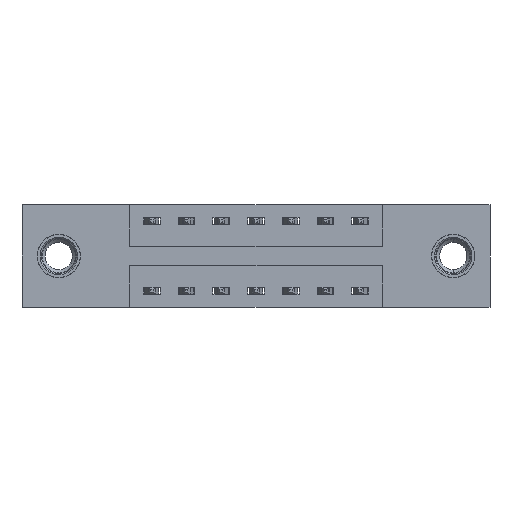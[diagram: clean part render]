
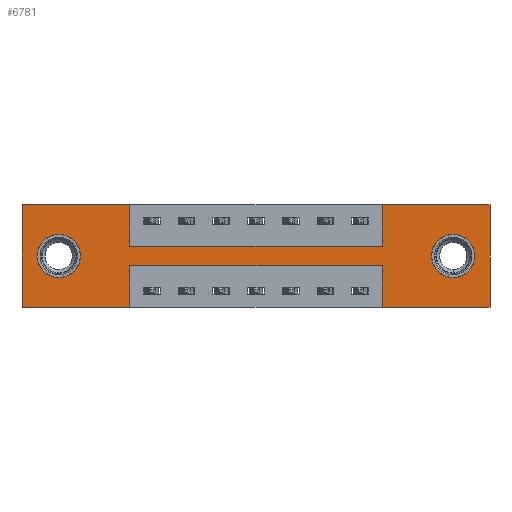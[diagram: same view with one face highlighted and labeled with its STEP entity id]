
A CAD part, front view. The second image highlights one B-rep face of the part: STEP entity #6781.
In plain terms, the highlighted planar face has unit normal (0, -1, 0).
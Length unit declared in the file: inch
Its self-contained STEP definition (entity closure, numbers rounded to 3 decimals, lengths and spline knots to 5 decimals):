
#21 = ORIENTED_EDGE ( 'NONE', *, *, #8824, .F. ) ;
#63 = VERTEX_POINT ( 'NONE', #7902 ) ;
#64 = LINE ( 'NONE', #4035, #4696 ) ;
#182 = CARTESIAN_POINT ( 'NONE',  ( 1.685, 0., 0. ) ) ;
#253 = CARTESIAN_POINT ( 'NONE',  ( 0., 0., 0. ) ) ;
#277 = CARTESIAN_POINT ( 'NONE',  ( 1.2975, 0., -0.15 ) ) ;
#473 = VECTOR ( 'NONE', #9578, 39.37008 ) ;
#514 = EDGE_LOOP ( 'NONE', ( #21, #2184, #2350, #3558, #3668, #4041, #4190, #4485, #4544, #4641, #4667, #4792 ) ) ;
#571 = VERTEX_POINT ( 'NONE', #4232 ) ;
#708 = DIRECTION ( 'NONE',  ( 0., 1., 0. ) ) ;
#737 = CARTESIAN_POINT ( 'NONE',  ( 0., 0., -0.37 ) ) ;
#781 = PLANE ( 'NONE',  #8333 ) ;
#822 = ORIENTED_EDGE ( 'NONE', *, *, #8264, .T. ) ;
#953 = VECTOR ( 'NONE', #6139, 39.37008 ) ;
#1035 = AXIS2_PLACEMENT_3D ( 'NONE', #7992, #3288, #8798 ) ;
#1152 = CARTESIAN_POINT ( 'NONE',  ( 1.2975, 0., -0.37 ) ) ;
#1377 = VECTOR ( 'NONE', #10301, 39.37008 ) ;
#1445 = ORIENTED_EDGE ( 'NONE', *, *, #5758, .T. ) ;
#1525 = CIRCLE ( 'NONE', #1035, 0.078 ) ;
#1699 = DIRECTION ( 'NONE',  ( 0., 0., -1. ) ) ;
#1819 = FACE_OUTER_BOUND ( 'NONE', #514, .T. ) ;
#1898 = AXIS2_PLACEMENT_3D ( 'NONE', #7675, #2993, #8492 ) ;
#2014 = VERTEX_POINT ( 'NONE', #2119 ) ;
#2034 = VERTEX_POINT ( 'NONE', #3030 ) ;
#2119 = CARTESIAN_POINT ( 'NONE',  ( 1.2975, 0., 0. ) ) ;
#2184 = ORIENTED_EDGE ( 'NONE', *, *, #10078, .F. ) ;
#2200 = CARTESIAN_POINT ( 'NONE',  ( 1.685, 0., 0. ) ) ;
#2203 = VECTOR ( 'NONE', #7014, 39.37008 ) ;
#2214 = LINE ( 'NONE', #182, #8295 ) ;
#2221 = CARTESIAN_POINT ( 'NONE',  ( 0.3875, 0., 0. ) ) ;
#2271 = CARTESIAN_POINT ( 'NONE',  ( 1.2975, 0., 0. ) ) ;
#2275 = DIRECTION ( 'NONE',  ( 0., 1., 0. ) ) ;
#2350 = ORIENTED_EDGE ( 'NONE', *, *, #10314, .F. ) ;
#2381 = CARTESIAN_POINT ( 'NONE',  ( 1.685, 0., -0.37 ) ) ;
#2468 = LINE ( 'NONE', #2271, #2203 ) ;
#2479 = VERTEX_POINT ( 'NONE', #9140 ) ;
#2491 = VERTEX_POINT ( 'NONE', #1152 ) ;
#2501 = EDGE_CURVE ( 'NONE', #5450, #2479, #2601, .T. ) ;
#2527 = ORIENTED_EDGE ( 'NONE', *, *, #3811, .T. ) ;
#2601 = LINE ( 'NONE', #8406, #8679 ) ;
#2859 = LINE ( 'NONE', #8814, #473 ) ;
#2993 = DIRECTION ( 'NONE',  ( 0., 1., 0. ) ) ;
#3030 = CARTESIAN_POINT ( 'NONE',  ( 1.5525, 0., -0.263 ) ) ;
#3065 = CARTESIAN_POINT ( 'NONE',  ( 0., 0., -0.37 ) ) ;
#3241 = EDGE_LOOP ( 'NONE', ( #1445, #7089 ) ) ;
#3265 = VERTEX_POINT ( 'NONE', #4670 ) ;
#3283 = CARTESIAN_POINT ( 'NONE',  ( 0.3875, 0., -0.37 ) ) ;
#3288 = DIRECTION ( 'NONE',  ( 0., 1., 0. ) ) ;
#3558 = ORIENTED_EDGE ( 'NONE', *, *, #8253, .F. ) ;
#3611 = VECTOR ( 'NONE', #9343, 39.37008 ) ;
#3668 = ORIENTED_EDGE ( 'NONE', *, *, #7835, .F. ) ;
#3706 = CIRCLE ( 'NONE', #9368, 0.078 ) ;
#3770 = FACE_BOUND ( 'NONE', #3241, .T. ) ;
#3811 = EDGE_CURVE ( 'NONE', #5606, #571, #8875, .T. ) ;
#3867 = VERTEX_POINT ( 'NONE', #9306 ) ;
#3914 = CARTESIAN_POINT ( 'NONE',  ( 0.3875, 0., -0.15 ) ) ;
#3962 = EDGE_CURVE ( 'NONE', #2034, #8661, #3706, .T. ) ;
#3999 = CARTESIAN_POINT ( 'NONE',  ( 1.5525, 0., -0.107 ) ) ;
#4035 = CARTESIAN_POINT ( 'NONE',  ( 0., 0., 0. ) ) ;
#4041 = ORIENTED_EDGE ( 'NONE', *, *, #9670, .F. ) ;
#4190 = ORIENTED_EDGE ( 'NONE', *, *, #8517, .F. ) ;
#4232 = CARTESIAN_POINT ( 'NONE',  ( 0.1325, 0., -0.107 ) ) ;
#4485 = ORIENTED_EDGE ( 'NONE', *, *, #7298, .F. ) ;
#4544 = ORIENTED_EDGE ( 'NONE', *, *, #7237, .F. ) ;
#4641 = ORIENTED_EDGE ( 'NONE', *, *, #5872, .F. ) ;
#4667 = ORIENTED_EDGE ( 'NONE', *, *, #2501, .F. ) ;
#4670 = CARTESIAN_POINT ( 'NONE',  ( 0.3875, 0., -0.15 ) ) ;
#4696 = VECTOR ( 'NONE', #10211, 39.37008 ) ;
#4733 = DIRECTION ( 'NONE',  ( 1., 0., 0. ) ) ;
#4792 = ORIENTED_EDGE ( 'NONE', *, *, #8117, .F. ) ;
#4965 = CARTESIAN_POINT ( 'NONE',  ( 0.3875, 0., 0. ) ) ;
#5442 = CIRCLE ( 'NONE', #6128, 0.078 ) ;
#5450 = VERTEX_POINT ( 'NONE', #6629 ) ;
#5606 = VERTEX_POINT ( 'NONE', #6816 ) ;
#5723 = CARTESIAN_POINT ( 'NONE',  ( 1.5525, 0., -0.185 ) ) ;
#5758 = EDGE_CURVE ( 'NONE', #8661, #2034, #5442, .T. ) ;
#5872 = EDGE_CURVE ( 'NONE', #2479, #10354, #64, .T. ) ;
#5883 = LINE ( 'NONE', #9533, #7654 ) ;
#5902 = VECTOR ( 'NONE', #4733, 39.37008 ) ;
#6005 = LINE ( 'NONE', #3065, #3611 ) ;
#6128 = AXIS2_PLACEMENT_3D ( 'NONE', #7016, #2275, #7826 ) ;
#6136 = LINE ( 'NONE', #2221, #8176 ) ;
#6139 = DIRECTION ( 'NONE',  ( 1., 0., 0. ) ) ;
#6462 = DIRECTION ( 'NONE',  ( 0., 0., -1. ) ) ;
#6519 = DIRECTION ( 'NONE',  ( 0., -1., 0. ) ) ;
#6629 = CARTESIAN_POINT ( 'NONE',  ( 0., 0., -0.37 ) ) ;
#6781 = ADVANCED_FACE ( 'NONE', ( #3770, #7945, #1819 ), #781, .T. ) ;
#6816 = CARTESIAN_POINT ( 'NONE',  ( 0.1325, 0., -0.263 ) ) ;
#7014 = DIRECTION ( 'NONE',  ( 0., 0., 1. ) ) ;
#7016 = CARTESIAN_POINT ( 'NONE',  ( 1.5525, 0., -0.185 ) ) ;
#7089 = ORIENTED_EDGE ( 'NONE', *, *, #3962, .T. ) ;
#7140 = DIRECTION ( 'NONE',  ( -1., 0., 0. ) ) ;
#7237 = EDGE_CURVE ( 'NONE', #10354, #3265, #6136, .T. ) ;
#7298 = EDGE_CURVE ( 'NONE', #3265, #7895, #9754, .T. ) ;
#7518 = LINE ( 'NONE', #3283, #1377 ) ;
#7654 = VECTOR ( 'NONE', #7140, 39.37008 ) ;
#7675 = CARTESIAN_POINT ( 'NONE',  ( 0.1325, 0., -0.185 ) ) ;
#7778 = VECTOR ( 'NONE', #10196, 39.37008 ) ;
#7826 = DIRECTION ( 'NONE',  ( 0., 0., -1. ) ) ;
#7835 = EDGE_CURVE ( 'NONE', #8459, #8677, #2214, .T. ) ;
#7895 = VERTEX_POINT ( 'NONE', #277 ) ;
#7902 = CARTESIAN_POINT ( 'NONE',  ( 1.2975, 0., -0.22 ) ) ;
#7945 = FACE_BOUND ( 'NONE', #10291, .T. ) ;
#7992 = CARTESIAN_POINT ( 'NONE',  ( 0.1325, 0., -0.185 ) ) ;
#8117 = EDGE_CURVE ( 'NONE', #9441, #5450, #6005, .T. ) ;
#8176 = VECTOR ( 'NONE', #10067, 39.37008 ) ;
#8253 = EDGE_CURVE ( 'NONE', #8677, #2491, #5883, .T. ) ;
#8264 = EDGE_CURVE ( 'NONE', #571, #5606, #1525, .T. ) ;
#8274 = LINE ( 'NONE', #9456, #7778 ) ;
#8295 = VECTOR ( 'NONE', #9212, 39.37008 ) ;
#8302 = CARTESIAN_POINT ( 'NONE',  ( 0.3875, 0., -0.37 ) ) ;
#8333 = AXIS2_PLACEMENT_3D ( 'NONE', #737, #6519, #1699 ) ;
#8406 = CARTESIAN_POINT ( 'NONE',  ( 0., 0., 0. ) ) ;
#8459 = VERTEX_POINT ( 'NONE', #2200 ) ;
#8492 = DIRECTION ( 'NONE',  ( 0., 0., 1. ) ) ;
#8517 = EDGE_CURVE ( 'NONE', #7895, #2014, #2468, .T. ) ;
#8661 = VERTEX_POINT ( 'NONE', #3999 ) ;
#8677 = VERTEX_POINT ( 'NONE', #2381 ) ;
#8679 = VECTOR ( 'NONE', #9202, 39.37008 ) ;
#8798 = DIRECTION ( 'NONE',  ( 0., 0., 1. ) ) ;
#8814 = CARTESIAN_POINT ( 'NONE',  ( 1.2975, 0., -0.37 ) ) ;
#8824 = EDGE_CURVE ( 'NONE', #3867, #9441, #7518, .T. ) ;
#8875 = CIRCLE ( 'NONE', #1898, 0.078 ) ;
#9028 = LINE ( 'NONE', #253, #953 ) ;
#9140 = CARTESIAN_POINT ( 'NONE',  ( 0., 0., 0. ) ) ;
#9202 = DIRECTION ( 'NONE',  ( 0., 0., 1. ) ) ;
#9212 = DIRECTION ( 'NONE',  ( 0., 0., -1. ) ) ;
#9306 = CARTESIAN_POINT ( 'NONE',  ( 0.3875, 0., -0.22 ) ) ;
#9343 = DIRECTION ( 'NONE',  ( -1., 0., 0. ) ) ;
#9368 = AXIS2_PLACEMENT_3D ( 'NONE', #5723, #708, #6462 ) ;
#9441 = VERTEX_POINT ( 'NONE', #8302 ) ;
#9456 = CARTESIAN_POINT ( 'NONE',  ( 0.3875, 0., -0.22 ) ) ;
#9533 = CARTESIAN_POINT ( 'NONE',  ( 0., 0., -0.37 ) ) ;
#9578 = DIRECTION ( 'NONE',  ( 0., 0., 1. ) ) ;
#9670 = EDGE_CURVE ( 'NONE', #2014, #8459, #9028, .T. ) ;
#9754 = LINE ( 'NONE', #3914, #5902 ) ;
#10067 = DIRECTION ( 'NONE',  ( 0., 0., -1. ) ) ;
#10078 = EDGE_CURVE ( 'NONE', #63, #3867, #8274, .T. ) ;
#10196 = DIRECTION ( 'NONE',  ( -1., 0., 0. ) ) ;
#10211 = DIRECTION ( 'NONE',  ( 1., 0., 0. ) ) ;
#10291 = EDGE_LOOP ( 'NONE', ( #822, #2527 ) ) ;
#10301 = DIRECTION ( 'NONE',  ( 0., 0., -1. ) ) ;
#10314 = EDGE_CURVE ( 'NONE', #2491, #63, #2859, .T. ) ;
#10354 = VERTEX_POINT ( 'NONE', #4965 ) ;
